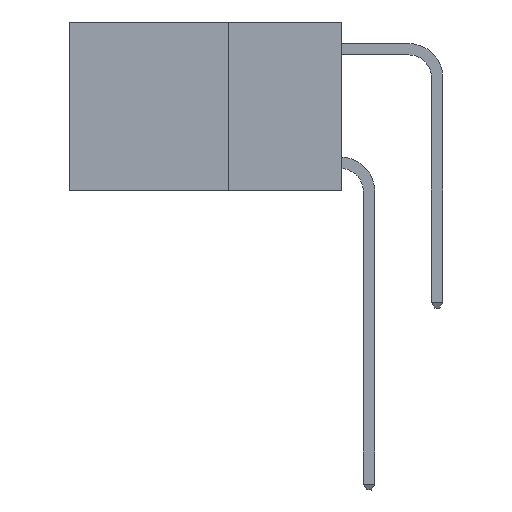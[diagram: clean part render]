
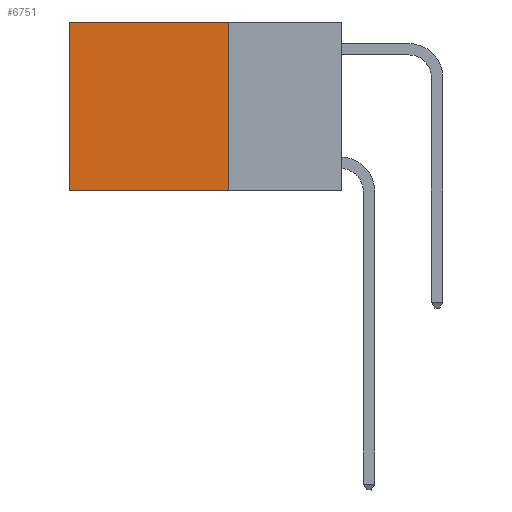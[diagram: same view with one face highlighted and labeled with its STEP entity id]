
A CAD part, left-side view. The second image highlights one B-rep face of the part: STEP entity #6751.
In plain terms, the highlighted planar face has unit normal (-1, 0, 0).
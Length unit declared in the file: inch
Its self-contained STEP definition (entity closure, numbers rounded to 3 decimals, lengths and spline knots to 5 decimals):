
#1042 = LINE ( 'NONE', #15891, #14529 ) ;
#1401 = ORIENTED_EDGE ( 'NONE', *, *, #19466, .T. ) ;
#1453 = CARTESIAN_POINT ( 'NONE',  ( 0.2625, 0.6, -0.37 ) ) ;
#1675 = CARTESIAN_POINT ( 'NONE',  ( 0.2625, 0.25, -0.37 ) ) ;
#3280 = AXIS2_PLACEMENT_3D ( 'NONE', #20993, #5623, #9141 ) ;
#3360 = DIRECTION ( 'NONE',  ( 0., 1., 0. ) ) ;
#3387 = VECTOR ( 'NONE', #3360, 39.37008 ) ;
#4007 = LINE ( 'NONE', #16118, #4263 ) ;
#4134 = VERTEX_POINT ( 'NONE', #18385 ) ;
#4263 = VECTOR ( 'NONE', #9178, 39.37008 ) ;
#5196 = FACE_OUTER_BOUND ( 'NONE', #18868, .T. ) ;
#5623 = DIRECTION ( 'NONE',  ( 1., 0., 0. ) ) ;
#6751 = ADVANCED_FACE ( 'NONE', ( #5196 ), #12415, .F. ) ;
#7800 = ORIENTED_EDGE ( 'NONE', *, *, #18739, .T. ) ;
#9141 = DIRECTION ( 'NONE',  ( 0., 0., -1. ) ) ;
#9151 = VERTEX_POINT ( 'NONE', #1453 ) ;
#9178 = DIRECTION ( 'NONE',  ( 0., 1., 0. ) ) ;
#9951 = EDGE_CURVE ( 'NONE', #4134, #20971, #18356, .T. ) ;
#9966 = CARTESIAN_POINT ( 'NONE',  ( 0.2625, 0.25, 0. ) ) ;
#11574 = VERTEX_POINT ( 'NONE', #12813 ) ;
#12094 = EDGE_CURVE ( 'NONE', #20971, #9151, #12383, .T. ) ;
#12383 = LINE ( 'NONE', #1675, #3387 ) ;
#12415 = PLANE ( 'NONE',  #3280 ) ;
#12813 = CARTESIAN_POINT ( 'NONE',  ( 0.2625, 0.6, 0. ) ) ;
#13316 = DIRECTION ( 'NONE',  ( 0., 0., -1. ) ) ;
#14529 = VECTOR ( 'NONE', #19319, 39.37008 ) ;
#15190 = ORIENTED_EDGE ( 'NONE', *, *, #9951, .F. ) ;
#15891 = CARTESIAN_POINT ( 'NONE',  ( 0.2625, 0.6, 0. ) ) ;
#16118 = CARTESIAN_POINT ( 'NONE',  ( 0.2625, 0.25, 0. ) ) ;
#16219 = VECTOR ( 'NONE', #13316, 39.37008 ) ;
#16976 = ORIENTED_EDGE ( 'NONE', *, *, #12094, .F. ) ;
#18356 = LINE ( 'NONE', #9966, #16219 ) ;
#18385 = CARTESIAN_POINT ( 'NONE',  ( 0.2625, 0.25, 0. ) ) ;
#18739 = EDGE_CURVE ( 'NONE', #4134, #11574, #4007, .T. ) ;
#18868 = EDGE_LOOP ( 'NONE', ( #1401, #16976, #15190, #7800 ) ) ;
#19319 = DIRECTION ( 'NONE',  ( 0., 0., -1. ) ) ;
#19466 = EDGE_CURVE ( 'NONE', #11574, #9151, #1042, .T. ) ;
#19525 = CARTESIAN_POINT ( 'NONE',  ( 0.2625, 0.25, -0.37 ) ) ;
#20971 = VERTEX_POINT ( 'NONE', #19525 ) ;
#20993 = CARTESIAN_POINT ( 'NONE',  ( 0.2625, 0.25, 0. ) ) ;
